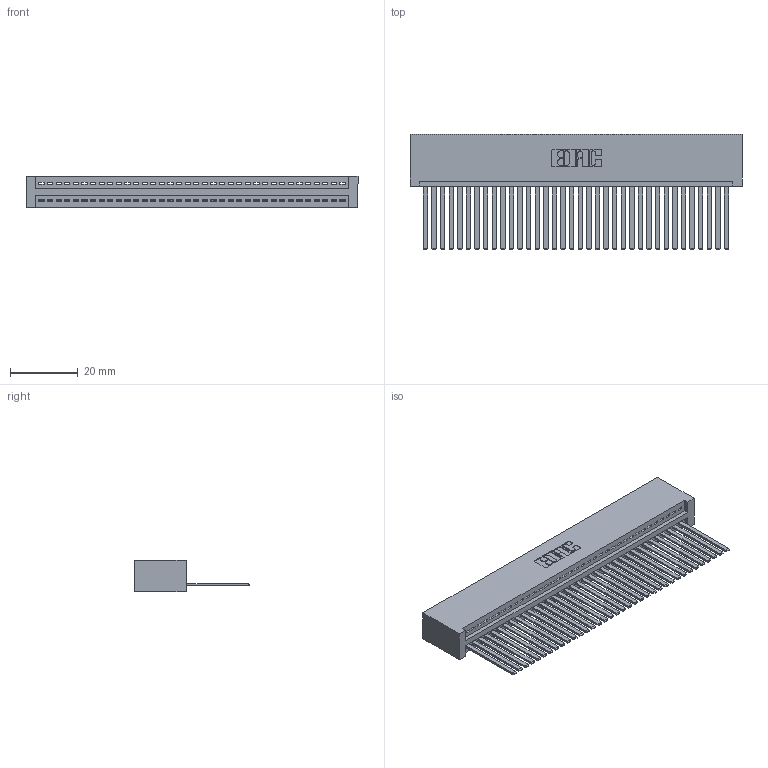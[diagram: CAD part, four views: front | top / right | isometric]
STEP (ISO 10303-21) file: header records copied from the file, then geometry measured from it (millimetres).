
FILE_DESCRIPTION (( 'STEP AP203' ), '1' );
FILE_NAME ('345-036-544-101.STEP', '2018-08-29T23:37:08', ( '' ), ( '' ), 'SwSTEP 2.0', 'SolidWorks 2016', '' );
FILE_SCHEMA (( 'CONFIG_CONTROL_DESIGN' ));
Length unit declared in the file: inch
Products named in the file (3): 345 Part_No Mounting Lugs; 345-292-001_345-293-144; 345-036-544-101
Assembly tree (37 placements, depth 2):
  345-036-544-101
    345 Part_No Mounting Lugs
    345-292-001_345-293-144  x36
Bounding box: 98.04 x 33.96 x 9.4 mm (x, y, z)
Volume: 10264.5 mm3; surface area: 15000.8 mm2
Topology: 37 solids, 37 shells, 1990 faces, 6005 edges, 3954 vertices
Faces by surface type: plane 1372, cylinder 618
Entity records: 27441 total; most frequent: CARTESIAN_POINT 4760, ORIENTED_EDGE 4730, DIRECTION 4157, EDGE_CURVE 2365, VECTOR 2101, LINE 2101, VERTEX_POINT 1574, AXIS2_PLACEMENT_3D 1028
